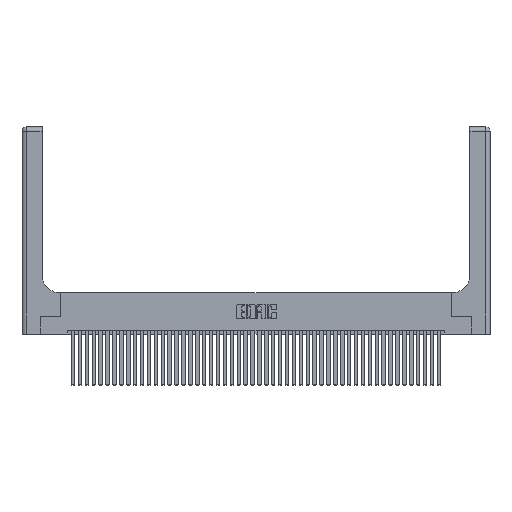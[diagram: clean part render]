
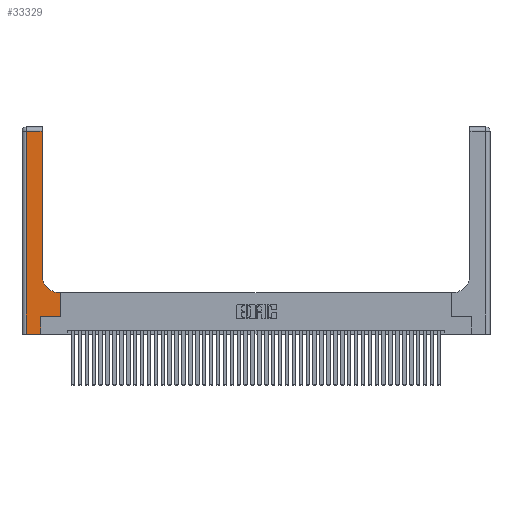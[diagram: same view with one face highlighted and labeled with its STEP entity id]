
A CAD part, top view. The second image highlights one B-rep face of the part: STEP entity #33329.
In plain terms, the highlighted planar face has unit normal (0, 0, 1).
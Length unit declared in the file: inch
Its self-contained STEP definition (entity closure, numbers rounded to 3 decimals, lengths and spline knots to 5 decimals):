
#424 = LINE ( 'NONE', #33299, #16420 ) ;
#793 = EDGE_CURVE ( 'NONE', #35460, #4777, #424, .T. ) ;
#1069 = EDGE_CURVE ( 'NONE', #31102, #17784, #20312, .T. ) ;
#2449 = VERTEX_POINT ( 'NONE', #22697 ) ;
#2558 = EDGE_CURVE ( 'NONE', #39627, #15215, #17943, .T. ) ;
#2649 = DIRECTION ( 'NONE',  ( 0., 1., 0. ) ) ;
#3238 = VECTOR ( 'NONE', #7436, 39.37008 ) ;
#3440 = VECTOR ( 'NONE', #33092, 39.37008 ) ;
#3623 = CARTESIAN_POINT ( 'NONE',  ( 0.5415, 0.6, 0.37 ) ) ;
#3949 = EDGE_LOOP ( 'NONE', ( #10325, #23921, #30135, #10680, #33774, #26145, #18505, #43924, #17771 ) ) ;
#4038 = AXIS2_PLACEMENT_3D ( 'NONE', #36163, #35849, #14610 ) ;
#4777 = VERTEX_POINT ( 'NONE', #14289 ) ;
#7436 = DIRECTION ( 'NONE',  ( 0., -1., 0. ) ) ;
#7604 = LINE ( 'NONE', #41856, #19224 ) ;
#7731 = DIRECTION ( 'NONE',  ( 1., 0., 0. ) ) ;
#8352 = AXIS2_PLACEMENT_3D ( 'NONE', #26905, #34014, #40663 ) ;
#9037 = EDGE_CURVE ( 'NONE', #2449, #31102, #15024, .T. ) ;
#9841 = LINE ( 'NONE', #10815, #3238 ) ;
#10143 = DIRECTION ( 'NONE',  ( 1., 0., 0. ) ) ;
#10325 = ORIENTED_EDGE ( 'NONE', *, *, #16655, .T. ) ;
#10680 = ORIENTED_EDGE ( 'NONE', *, *, #19194, .T. ) ;
#10815 = CARTESIAN_POINT ( 'NONE',  ( 0.06, 3., 0.37 ) ) ;
#11436 = VECTOR ( 'NONE', #15612, 39.37008 ) ;
#13739 = CARTESIAN_POINT ( 'NONE',  ( 0.2915, 0.6, 0.37 ) ) ;
#14289 = CARTESIAN_POINT ( 'NONE',  ( 0.269, 0.25, 0.37 ) ) ;
#14610 = DIRECTION ( 'NONE',  ( -1., 0., 0. ) ) ;
#15002 = LINE ( 'NONE', #40355, #3440 ) ;
#15024 = LINE ( 'NONE', #34182, #38829 ) ;
#15215 = VERTEX_POINT ( 'NONE', #31481 ) ;
#15612 = DIRECTION ( 'NONE',  ( -1., 0., 0. ) ) ;
#16227 = CARTESIAN_POINT ( 'NONE',  ( 0.5585, 0.6, 0.37 ) ) ;
#16286 = VECTOR ( 'NONE', #45211, 39.37008 ) ;
#16420 = VECTOR ( 'NONE', #43636, 39.37008 ) ;
#16655 = EDGE_CURVE ( 'NONE', #17671, #39627, #15002, .T. ) ;
#17671 = VERTEX_POINT ( 'NONE', #24951 ) ;
#17771 = ORIENTED_EDGE ( 'NONE', *, *, #26877, .T. ) ;
#17784 = VERTEX_POINT ( 'NONE', #3623 ) ;
#17943 = LINE ( 'NONE', #31742, #16286 ) ;
#18505 = ORIENTED_EDGE ( 'NONE', *, *, #9037, .T. ) ;
#19194 = EDGE_CURVE ( 'NONE', #40627, #35460, #30353, .T. ) ;
#19202 = EDGE_CURVE ( 'NONE', #15215, #40627, #9841, .T. ) ;
#19224 = VECTOR ( 'NONE', #10143, 39.37008 ) ;
#20312 = LINE ( 'NONE', #13739, #11436 ) ;
#22596 = VECTOR ( 'NONE', #7731, 39.37008 ) ;
#22697 = CARTESIAN_POINT ( 'NONE',  ( 0.5585, 0.25, 0.37 ) ) ;
#23921 = ORIENTED_EDGE ( 'NONE', *, *, #2558, .T. ) ;
#24951 = CARTESIAN_POINT ( 'NONE',  ( 0.2915, 0.85, 0.37 ) ) ;
#25356 = PLANE ( 'NONE',  #4038 ) ;
#26145 = ORIENTED_EDGE ( 'NONE', *, *, #39603, .T. ) ;
#26877 = EDGE_CURVE ( 'NONE', #17784, #17671, #36418, .T. ) ;
#26905 = CARTESIAN_POINT ( 'NONE',  ( 0.5415, 0.85, 0.37 ) ) ;
#28768 = CARTESIAN_POINT ( 'NONE',  ( 0., 0., 0.37 ) ) ;
#30058 = CARTESIAN_POINT ( 'NONE',  ( 0.269, 0., 0.37 ) ) ;
#30135 = ORIENTED_EDGE ( 'NONE', *, *, #19202, .T. ) ;
#30353 = LINE ( 'NONE', #28768, #22596 ) ;
#30362 = FACE_OUTER_BOUND ( 'NONE', #3949, .T. ) ;
#31102 = VERTEX_POINT ( 'NONE', #16227 ) ;
#31481 = CARTESIAN_POINT ( 'NONE',  ( 0.06, 2.94, 0.37 ) ) ;
#31742 = CARTESIAN_POINT ( 'NONE',  ( 0., 2.94, 0.37 ) ) ;
#33092 = DIRECTION ( 'NONE',  ( 0., 1., 0. ) ) ;
#33299 = CARTESIAN_POINT ( 'NONE',  ( 0.269, 0., 0.37 ) ) ;
#33329 = ADVANCED_FACE ( 'NONE', ( #30362 ), #25356, .F. ) ;
#33532 = CARTESIAN_POINT ( 'NONE',  ( 0.06, 0., 0.37 ) ) ;
#33774 = ORIENTED_EDGE ( 'NONE', *, *, #793, .T. ) ;
#34014 = DIRECTION ( 'NONE',  ( 0., 0., -1. ) ) ;
#34182 = CARTESIAN_POINT ( 'NONE',  ( 0.5585, 0.25, 0.37 ) ) ;
#35460 = VERTEX_POINT ( 'NONE', #30058 ) ;
#35849 = DIRECTION ( 'NONE',  ( 0., 0., -1. ) ) ;
#36163 = CARTESIAN_POINT ( 'NONE',  ( 0., 3., 0.37 ) ) ;
#36418 = CIRCLE ( 'NONE', #8352, 0.25 ) ;
#38428 = CARTESIAN_POINT ( 'NONE',  ( 0.2915, 2.94, 0.37 ) ) ;
#38829 = VECTOR ( 'NONE', #2649, 39.37008 ) ;
#39603 = EDGE_CURVE ( 'NONE', #4777, #2449, #7604, .T. ) ;
#39627 = VERTEX_POINT ( 'NONE', #38428 ) ;
#40355 = CARTESIAN_POINT ( 'NONE',  ( 0.2915, 3., 0.37 ) ) ;
#40627 = VERTEX_POINT ( 'NONE', #33532 ) ;
#40663 = DIRECTION ( 'NONE',  ( 1., 0., 0. ) ) ;
#41856 = CARTESIAN_POINT ( 'NONE',  ( 0.269, 0.25, 0.37 ) ) ;
#43636 = DIRECTION ( 'NONE',  ( 0., 1., 0. ) ) ;
#43924 = ORIENTED_EDGE ( 'NONE', *, *, #1069, .T. ) ;
#45211 = DIRECTION ( 'NONE',  ( -1., 0., 0. ) ) ;
